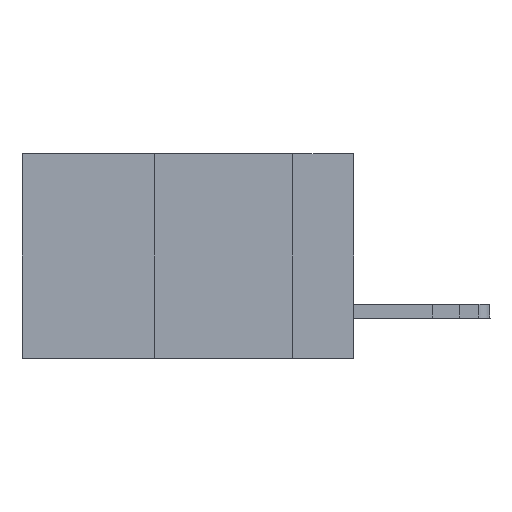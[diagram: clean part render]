
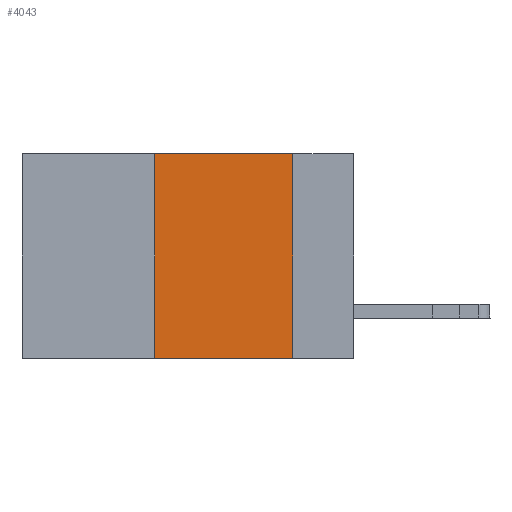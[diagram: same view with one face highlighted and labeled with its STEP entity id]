
A CAD part, left-side view. The second image highlights one B-rep face of the part: STEP entity #4043.
In plain terms, the highlighted planar face has unit normal (-1, 0, 0).
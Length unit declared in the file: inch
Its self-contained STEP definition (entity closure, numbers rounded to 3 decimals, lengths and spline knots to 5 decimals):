
#217 = DIRECTION ( 'NONE',  ( 1., 0., 0. ) ) ;
#623 = LINE ( 'NONE', #2667, #15797 ) ;
#825 = CARTESIAN_POINT ( 'NONE',  ( 0., 0.6, 0. ) ) ;
#2667 = CARTESIAN_POINT ( 'NONE',  ( 0., 0.36, 0. ) ) ;
#3460 = FACE_OUTER_BOUND ( 'NONE', #8359, .T. ) ;
#3477 = VECTOR ( 'NONE', #9376, 39.37008 ) ;
#4015 = CARTESIAN_POINT ( 'NONE',  ( 0., 0.6, -0.37 ) ) ;
#4043 = ADVANCED_FACE ( 'NONE', ( #3460 ), #15348, .F. ) ;
#5005 = VERTEX_POINT ( 'NONE', #16556 ) ;
#6456 = EDGE_CURVE ( 'NONE', #5005, #18620, #12305, .T. ) ;
#6615 = VERTEX_POINT ( 'NONE', #7045 ) ;
#6730 = CARTESIAN_POINT ( 'NONE',  ( 0., 0.11, 0. ) ) ;
#6920 = VERTEX_POINT ( 'NONE', #16709 ) ;
#7045 = CARTESIAN_POINT ( 'NONE',  ( 0., 0.11, -0.37 ) ) ;
#7119 = AXIS2_PLACEMENT_3D ( 'NONE', #9262, #217, #15954 ) ;
#7705 = CARTESIAN_POINT ( 'NONE',  ( 0., 0.11, 0. ) ) ;
#7786 = LINE ( 'NONE', #4015, #15986 ) ;
#8359 = EDGE_LOOP ( 'NONE', ( #11149, #17122, #10786, #17882 ) ) ;
#8496 = LINE ( 'NONE', #6730, #11452 ) ;
#9262 = CARTESIAN_POINT ( 'NONE',  ( 0., 0.6, 0. ) ) ;
#9376 = DIRECTION ( 'NONE',  ( 0., -1., 0. ) ) ;
#10786 = ORIENTED_EDGE ( 'NONE', *, *, #11303, .F. ) ;
#11149 = ORIENTED_EDGE ( 'NONE', *, *, #13814, .F. ) ;
#11303 = EDGE_CURVE ( 'NONE', #6920, #5005, #623, .T. ) ;
#11452 = VECTOR ( 'NONE', #18318, 39.37008 ) ;
#12305 = LINE ( 'NONE', #825, #3477 ) ;
#13814 = EDGE_CURVE ( 'NONE', #18620, #6615, #8496, .T. ) ;
#14064 = DIRECTION ( 'NONE',  ( 0., -1., 0. ) ) ;
#14251 = DIRECTION ( 'NONE',  ( 0., 0., 1. ) ) ;
#14541 = EDGE_CURVE ( 'NONE', #6920, #6615, #7786, .T. ) ;
#15348 = PLANE ( 'NONE',  #7119 ) ;
#15797 = VECTOR ( 'NONE', #14251, 39.37008 ) ;
#15954 = DIRECTION ( 'NONE',  ( 0., 0., -1. ) ) ;
#15986 = VECTOR ( 'NONE', #14064, 39.37008 ) ;
#16556 = CARTESIAN_POINT ( 'NONE',  ( 0., 0.36, 0. ) ) ;
#16709 = CARTESIAN_POINT ( 'NONE',  ( 0., 0.36, -0.37 ) ) ;
#17122 = ORIENTED_EDGE ( 'NONE', *, *, #6456, .F. ) ;
#17882 = ORIENTED_EDGE ( 'NONE', *, *, #14541, .T. ) ;
#18318 = DIRECTION ( 'NONE',  ( 0., 0., -1. ) ) ;
#18620 = VERTEX_POINT ( 'NONE', #7705 ) ;
